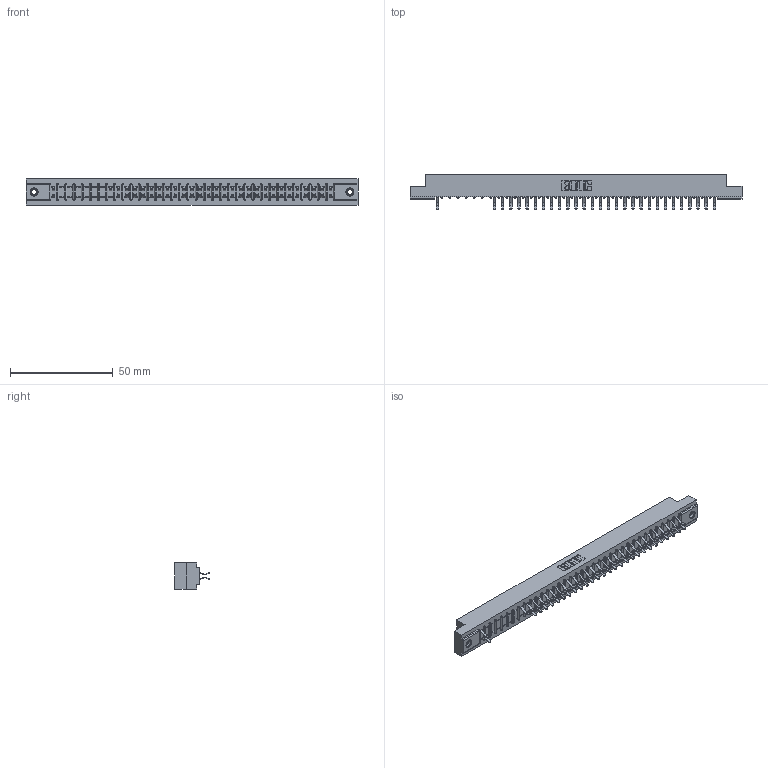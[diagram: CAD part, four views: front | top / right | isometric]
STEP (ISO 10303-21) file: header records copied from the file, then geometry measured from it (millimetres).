
FILE_DESCRIPTION (( 'STEP AP203' ), '1' );
FILE_NAME ('307-070-556-207.STEP', '2018-08-06T13:15:07', ( '' ), ( '' ), 'SwSTEP 2.0', 'SolidWorks 2016', '' );
FILE_SCHEMA (( 'CONFIG_CONTROL_DESIGN' ));
Length unit declared in the file: inch
Products named in the file (4): 345-250-001_345-250-005-103; 307-070-556-207; 307 Part_.156 Dia Mounting Holes; 307-290-001_556
Assembly tree (60 placements, depth 2):
  307-070-556-207
    307 Part_.156 Dia Mounting Holes
    307-290-001_556  x57
    345-250-001_345-250-005-103  x2
Bounding box: 161.7 x 16.97 x 12.7 mm (x, y, z)
Volume: 16952.7 mm3; surface area: 19379.2 mm2
Topology: 60 solids, 60 shells, 3194 faces, 8969 edges, 5798 vertices
Faces by surface type: plane 2061, cylinder 1045, sphere 72, cone 12, torus 4
Entity records: 32861 total; most frequent: CARTESIAN_POINT 5417, ORIENTED_EDGE 5374, DIRECTION 5305, EDGE_CURVE 2687, VECTOR 2057, LINE 2057, VERTEX_POINT 1736, AXIS2_PLACEMENT_3D 1624
